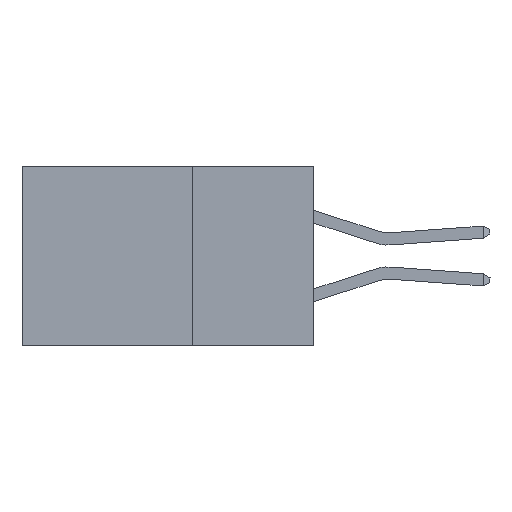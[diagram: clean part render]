
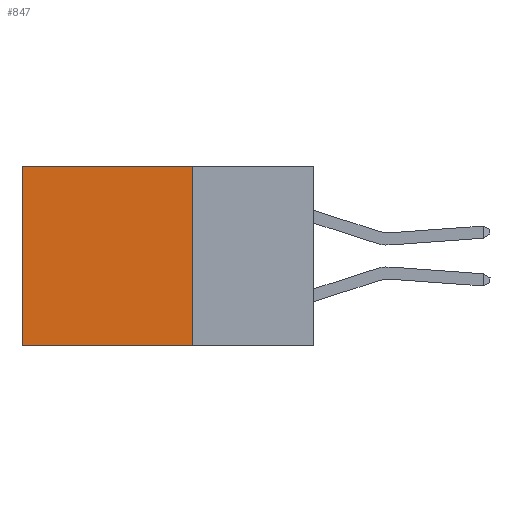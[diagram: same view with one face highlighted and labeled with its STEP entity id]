
A CAD part, left-side view. The second image highlights one B-rep face of the part: STEP entity #847.
In plain terms, the highlighted planar face has unit normal (-1, 0, 0).
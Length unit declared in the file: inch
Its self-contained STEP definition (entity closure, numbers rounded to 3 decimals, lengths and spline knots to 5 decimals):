
#207 = CARTESIAN_POINT ( 'NONE',  ( 0.2875, 0.25, -0.37 ) ) ;
#847 = ADVANCED_FACE ( 'NONE', ( #9021 ), #11978, .F. ) ;
#2160 = DIRECTION ( 'NONE',  ( 0., 1., 0. ) ) ;
#2730 = DIRECTION ( 'NONE',  ( 0., 0., -1. ) ) ;
#2876 = LINE ( 'NONE', #9451, #17031 ) ;
#5631 = VERTEX_POINT ( 'NONE', #16571 ) ;
#5852 = LINE ( 'NONE', #207, #10768 ) ;
#6173 = ORIENTED_EDGE ( 'NONE', *, *, #18731, .F. ) ;
#6357 = CARTESIAN_POINT ( 'NONE',  ( 0.2875, 0.6, 0. ) ) ;
#7755 = CARTESIAN_POINT ( 'NONE',  ( 0.2875, 0.25, 0. ) ) ;
#8125 = VECTOR ( 'NONE', #16752, 39.37008 ) ;
#8157 = EDGE_LOOP ( 'NONE', ( #19908, #6173, #15753, #10824 ) ) ;
#9021 = FACE_OUTER_BOUND ( 'NONE', #8157, .T. ) ;
#9451 = CARTESIAN_POINT ( 'NONE',  ( 0.2875, 0.25, 0. ) ) ;
#10663 = VECTOR ( 'NONE', #2160, 39.37008 ) ;
#10768 = VECTOR ( 'NONE', #11227, 39.37008 ) ;
#10824 = ORIENTED_EDGE ( 'NONE', *, *, #14591, .T. ) ;
#11227 = DIRECTION ( 'NONE',  ( 0., 1., 0. ) ) ;
#11314 = VERTEX_POINT ( 'NONE', #6357 ) ;
#11341 = DIRECTION ( 'NONE',  ( 0., 0., -1. ) ) ;
#11978 = PLANE ( 'NONE',  #23064 ) ;
#13115 = VERTEX_POINT ( 'NONE', #21926 ) ;
#13855 = DIRECTION ( 'NONE',  ( 1., 0., 0. ) ) ;
#14591 = EDGE_CURVE ( 'NONE', #13115, #11314, #20414, .T. ) ;
#14950 = CARTESIAN_POINT ( 'NONE',  ( 0.2875, 0.6, 0. ) ) ;
#15753 = ORIENTED_EDGE ( 'NONE', *, *, #20026, .F. ) ;
#16035 = VERTEX_POINT ( 'NONE', #20807 ) ;
#16571 = CARTESIAN_POINT ( 'NONE',  ( 0.2875, 0.6, -0.37 ) ) ;
#16752 = DIRECTION ( 'NONE',  ( 0., 0., -1. ) ) ;
#17031 = VECTOR ( 'NONE', #11341, 39.37008 ) ;
#18731 = EDGE_CURVE ( 'NONE', #16035, #5631, #5852, .T. ) ;
#19225 = CARTESIAN_POINT ( 'NONE',  ( 0.2875, 0.25, 0. ) ) ;
#19322 = EDGE_CURVE ( 'NONE', #11314, #5631, #22739, .T. ) ;
#19908 = ORIENTED_EDGE ( 'NONE', *, *, #19322, .T. ) ;
#20026 = EDGE_CURVE ( 'NONE', #13115, #16035, #2876, .T. ) ;
#20414 = LINE ( 'NONE', #7755, #10663 ) ;
#20807 = CARTESIAN_POINT ( 'NONE',  ( 0.2875, 0.25, -0.37 ) ) ;
#21926 = CARTESIAN_POINT ( 'NONE',  ( 0.2875, 0.25, 0. ) ) ;
#22739 = LINE ( 'NONE', #14950, #8125 ) ;
#23064 = AXIS2_PLACEMENT_3D ( 'NONE', #19225, #13855, #2730 ) ;
